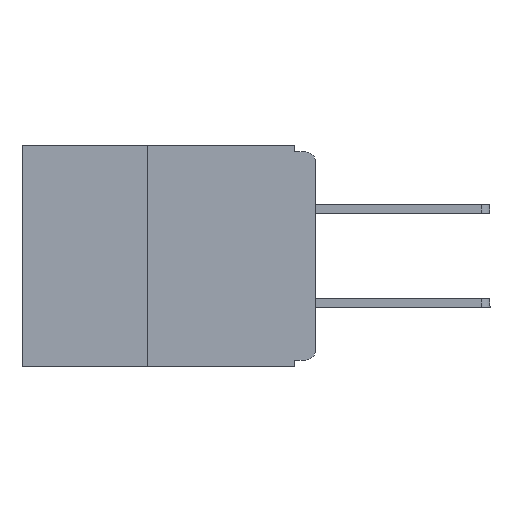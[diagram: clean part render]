
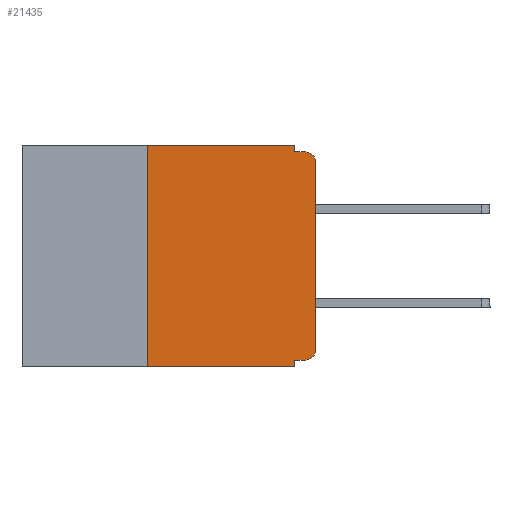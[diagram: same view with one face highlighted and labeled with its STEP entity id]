
A CAD part, left-side view. The second image highlights one B-rep face of the part: STEP entity #21435.
In plain terms, the highlighted planar face has unit normal (-1, 0, 0).
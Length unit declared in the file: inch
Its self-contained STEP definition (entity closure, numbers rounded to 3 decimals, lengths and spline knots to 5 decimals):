
#428 = ORIENTED_EDGE ( 'NONE', *, *, #13549, .F. ) ;
#551 = ORIENTED_EDGE ( 'NONE', *, *, #2730, .T. ) ;
#845 = VERTEX_POINT ( 'NONE', #7010 ) ;
#1787 = CARTESIAN_POINT ( 'NONE',  ( 0., 0.031, 0. ) ) ;
#1839 = CIRCLE ( 'NONE', #20158, 0.015 ) ;
#1984 = VECTOR ( 'NONE', #26139, 39.37008 ) ;
#2056 = VERTEX_POINT ( 'NONE', #25730 ) ;
#2059 = CARTESIAN_POINT ( 'NONE',  ( 0., 0.437, -0.33 ) ) ;
#2627 = CARTESIAN_POINT ( 'NONE',  ( 0., 0.031, -0.32 ) ) ;
#2666 = VECTOR ( 'NONE', #26414, 39.37008 ) ;
#2730 = EDGE_CURVE ( 'NONE', #20670, #25374, #1839, .T. ) ;
#3199 = VERTEX_POINT ( 'NONE', #14158 ) ;
#3418 = PLANE ( 'NONE',  #24816 ) ;
#3523 = VERTEX_POINT ( 'NONE', #22474 ) ;
#3694 = CARTESIAN_POINT ( 'NONE',  ( 0., 0., -0.025 ) ) ;
#3736 = CARTESIAN_POINT ( 'NONE',  ( 0., 0., -0.01 ) ) ;
#4076 = DIRECTION ( 'NONE',  ( 0., -1., 0. ) ) ;
#4413 = CARTESIAN_POINT ( 'NONE',  ( 0., 0.031, -0.33 ) ) ;
#4919 = DIRECTION ( 'NONE',  ( -1., 0., 0. ) ) ;
#6173 = CARTESIAN_POINT ( 'NONE',  ( 0., 0.25, -0.33 ) ) ;
#6275 = CARTESIAN_POINT ( 'NONE',  ( 0., 0., -0.32 ) ) ;
#6524 = FACE_OUTER_BOUND ( 'NONE', #11811, .T. ) ;
#6543 = CARTESIAN_POINT ( 'NONE',  ( 0., 0.25, -0.33 ) ) ;
#6553 = EDGE_CURVE ( 'NONE', #3523, #845, #11376, .T. ) ;
#6636 = DIRECTION ( 'NONE',  ( 0., -1., 0. ) ) ;
#6693 = EDGE_CURVE ( 'NONE', #11088, #3199, #13612, .T. ) ;
#6709 = EDGE_CURVE ( 'NONE', #25374, #15665, #18492, .T. ) ;
#6798 = CARTESIAN_POINT ( 'NONE',  ( 0., 0., -0.305 ) ) ;
#7010 = CARTESIAN_POINT ( 'NONE',  ( 0., 0.015, -0.01 ) ) ;
#7927 = ORIENTED_EDGE ( 'NONE', *, *, #6709, .T. ) ;
#8285 = DIRECTION ( 'NONE',  ( 0., 1., 0. ) ) ;
#8430 = VECTOR ( 'NONE', #14191, 39.37008 ) ;
#8476 = VERTEX_POINT ( 'NONE', #2627 ) ;
#9054 = LINE ( 'NONE', #1787, #8430 ) ;
#9353 = LINE ( 'NONE', #18975, #19717 ) ;
#10119 = VERTEX_POINT ( 'NONE', #12219 ) ;
#10513 = ORIENTED_EDGE ( 'NONE', *, *, #6693, .T. ) ;
#10991 = ORIENTED_EDGE ( 'NONE', *, *, #25207, .F. ) ;
#11088 = VERTEX_POINT ( 'NONE', #6543 ) ;
#11224 = VECTOR ( 'NONE', #14723, 39.37008 ) ;
#11346 = ORIENTED_EDGE ( 'NONE', *, *, #6553, .F. ) ;
#11376 = LINE ( 'NONE', #3736, #16907 ) ;
#11712 = DIRECTION ( 'NONE',  ( 0., 0., -1. ) ) ;
#11811 = EDGE_LOOP ( 'NONE', ( #7927, #13283, #11346, #12609, #12368, #12136, #10513, #428, #10991, #551 ) ) ;
#11867 = LINE ( 'NONE', #4413, #11224 ) ;
#12025 = VECTOR ( 'NONE', #18509, 39.37008 ) ;
#12136 = ORIENTED_EDGE ( 'NONE', *, *, #26209, .F. ) ;
#12219 = CARTESIAN_POINT ( 'NONE',  ( 0., 0.031, 0. ) ) ;
#12368 = ORIENTED_EDGE ( 'NONE', *, *, #21123, .F. ) ;
#12609 = ORIENTED_EDGE ( 'NONE', *, *, #20936, .F. ) ;
#13283 = ORIENTED_EDGE ( 'NONE', *, *, #20611, .T. ) ;
#13549 = EDGE_CURVE ( 'NONE', #8476, #3199, #11867, .T. ) ;
#13612 = LINE ( 'NONE', #2059, #2666 ) ;
#14158 = CARTESIAN_POINT ( 'NONE',  ( 0., 0.031, -0.33 ) ) ;
#14191 = DIRECTION ( 'NONE',  ( 0., 0., -1. ) ) ;
#14723 = DIRECTION ( 'NONE',  ( 0., 0., -1. ) ) ;
#15665 = VERTEX_POINT ( 'NONE', #3694 ) ;
#15836 = CARTESIAN_POINT ( 'NONE',  ( 0., 0.437, 0. ) ) ;
#16907 = VECTOR ( 'NONE', #4076, 39.37008 ) ;
#17313 = CARTESIAN_POINT ( 'NONE',  ( 0., 0.015, -0.025 ) ) ;
#17560 = LINE ( 'NONE', #6173, #12025 ) ;
#18261 = LINE ( 'NONE', #6275, #22934 ) ;
#18492 = LINE ( 'NONE', #26175, #1984 ) ;
#18509 = DIRECTION ( 'NONE',  ( 0., 0., 1. ) ) ;
#18975 = CARTESIAN_POINT ( 'NONE',  ( 0., 0.437, 0. ) ) ;
#19337 = DIRECTION ( 'NONE',  ( 0., 0., -1. ) ) ;
#19421 = CARTESIAN_POINT ( 'NONE',  ( 0., 0.015, -0.32 ) ) ;
#19717 = VECTOR ( 'NONE', #6636, 39.37008 ) ;
#20158 = AXIS2_PLACEMENT_3D ( 'NONE', #20988, #21734, #22189 ) ;
#20420 = CIRCLE ( 'NONE', #23616, 0.015 ) ;
#20611 = EDGE_CURVE ( 'NONE', #15665, #845, #20420, .T. ) ;
#20670 = VERTEX_POINT ( 'NONE', #19421 ) ;
#20936 = EDGE_CURVE ( 'NONE', #10119, #3523, #9054, .T. ) ;
#20988 = CARTESIAN_POINT ( 'NONE',  ( 0., 0.015, -0.305 ) ) ;
#21123 = EDGE_CURVE ( 'NONE', #2056, #10119, #9353, .T. ) ;
#21435 = ADVANCED_FACE ( 'NONE', ( #6524 ), #3418, .F. ) ;
#21734 = DIRECTION ( 'NONE',  ( -1., 0., 0. ) ) ;
#22189 = DIRECTION ( 'NONE',  ( 0., 0., -1. ) ) ;
#22474 = CARTESIAN_POINT ( 'NONE',  ( 0., 0.031, -0.01 ) ) ;
#22934 = VECTOR ( 'NONE', #8285, 39.37008 ) ;
#23616 = AXIS2_PLACEMENT_3D ( 'NONE', #17313, #4919, #19337 ) ;
#23880 = DIRECTION ( 'NONE',  ( 1., 0., 0. ) ) ;
#24816 = AXIS2_PLACEMENT_3D ( 'NONE', #15836, #23880, #11712 ) ;
#25207 = EDGE_CURVE ( 'NONE', #20670, #8476, #18261, .T. ) ;
#25374 = VERTEX_POINT ( 'NONE', #6798 ) ;
#25730 = CARTESIAN_POINT ( 'NONE',  ( 0., 0.25, 0. ) ) ;
#26139 = DIRECTION ( 'NONE',  ( 0., 0., 1. ) ) ;
#26175 = CARTESIAN_POINT ( 'NONE',  ( 0., 0., 0. ) ) ;
#26209 = EDGE_CURVE ( 'NONE', #11088, #2056, #17560, .T. ) ;
#26414 = DIRECTION ( 'NONE',  ( 0., -1., 0. ) ) ;
